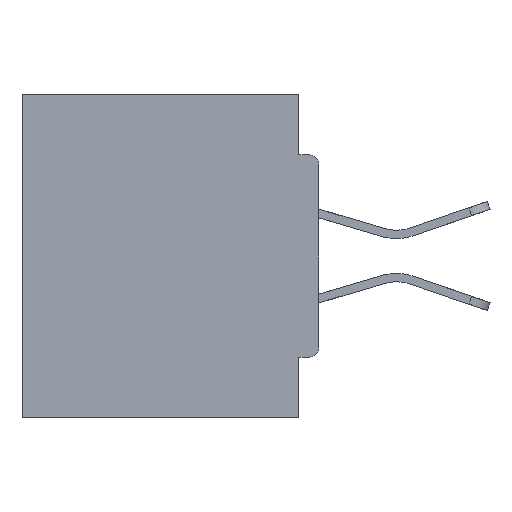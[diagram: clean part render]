
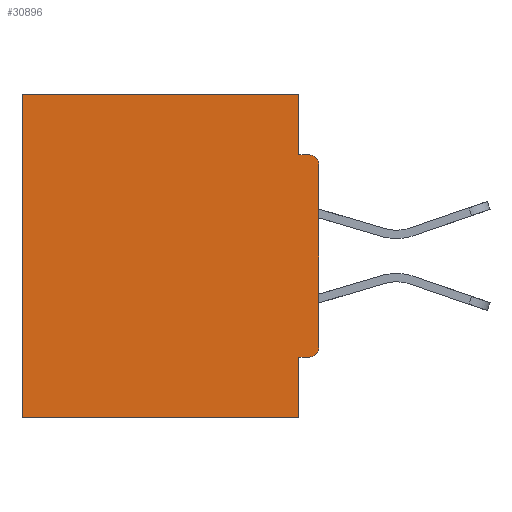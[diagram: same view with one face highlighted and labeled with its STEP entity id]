
A CAD part, left-side view. The second image highlights one B-rep face of the part: STEP entity #30896.
In plain terms, the highlighted planar face has unit normal (-1, 0, 0).
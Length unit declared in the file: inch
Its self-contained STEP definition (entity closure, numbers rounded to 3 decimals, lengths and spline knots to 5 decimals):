
#879 = EDGE_CURVE ( 'NONE', #28704, #24435, #10681, .T. ) ;
#1654 = EDGE_CURVE ( 'NONE', #22127, #19679, #16841, .T. ) ;
#3004 = ORIENTED_EDGE ( 'NONE', *, *, #30974, .F. ) ;
#3491 = DIRECTION ( 'NONE',  ( 0., 0., -1. ) ) ;
#3579 = DIRECTION ( 'NONE',  ( 0., 0., -1. ) ) ;
#3923 = CARTESIAN_POINT ( 'NONE',  ( 0.298, 0.031, -0.5 ) ) ;
#4585 = EDGE_CURVE ( 'NONE', #12120, #24927, #23704, .T. ) ;
#4596 = DIRECTION ( 'NONE',  ( 0., 1., 0. ) ) ;
#5029 = CARTESIAN_POINT ( 'NONE',  ( 0.298, 0.031, -0.5 ) ) ;
#5645 = EDGE_CURVE ( 'NONE', #28704, #21075, #11145, .T. ) ;
#5702 = CARTESIAN_POINT ( 'NONE',  ( 0.298, 0., -0.0935 ) ) ;
#5826 = ORIENTED_EDGE ( 'NONE', *, *, #1654, .F. ) ;
#6322 = CARTESIAN_POINT ( 'NONE',  ( 0.298, 0.031, -0.5 ) ) ;
#6700 = CARTESIAN_POINT ( 'NONE',  ( 0.298, 0., -0.4065 ) ) ;
#6781 = ORIENTED_EDGE ( 'NONE', *, *, #25753, .T. ) ;
#6851 = CARTESIAN_POINT ( 'NONE',  ( 0.298, 0.031, -0.0935 ) ) ;
#6872 = EDGE_CURVE ( 'NONE', #12120, #23094, #12220, .T. ) ;
#6971 = LINE ( 'NONE', #25047, #19478 ) ;
#7345 = DIRECTION ( 'NONE',  ( 0., 0., -1. ) ) ;
#7388 = LINE ( 'NONE', #5702, #29672 ) ;
#7555 = CARTESIAN_POINT ( 'NONE',  ( 0.298, 0.015, -0.4065 ) ) ;
#7778 = DIRECTION ( 'NONE',  ( 0., -1., 0. ) ) ;
#8684 = PLANE ( 'NONE',  #21706 ) ;
#9737 = AXIS2_PLACEMENT_3D ( 'NONE', #18416, #30878, #3491 ) ;
#9887 = VECTOR ( 'NONE', #28281, 39.37008 ) ;
#10078 = CARTESIAN_POINT ( 'NONE',  ( 0.298, 0., -0.1085 ) ) ;
#10387 = CARTESIAN_POINT ( 'NONE',  ( 0.298, 0., 0. ) ) ;
#10681 = LINE ( 'NONE', #10387, #9887 ) ;
#10972 = DIRECTION ( 'NONE',  ( 1., 0., 0. ) ) ;
#11043 = VECTOR ( 'NONE', #21383, 39.37008 ) ;
#11145 = CIRCLE ( 'NONE', #28000, 0.015 ) ;
#12120 = VERTEX_POINT ( 'NONE', #28115 ) ;
#12220 = LINE ( 'NONE', #3923, #11043 ) ;
#12243 = CARTESIAN_POINT ( 'NONE',  ( 0.298, 0.015, -0.1085 ) ) ;
#13390 = CARTESIAN_POINT ( 'NONE',  ( 0.298, 0., 0. ) ) ;
#14209 = ORIENTED_EDGE ( 'NONE', *, *, #5645, .T. ) ;
#15392 = VECTOR ( 'NONE', #3579, 39.37008 ) ;
#15885 = CARTESIAN_POINT ( 'NONE',  ( 0.298, 0.015, -0.0935 ) ) ;
#16770 = CARTESIAN_POINT ( 'NONE',  ( 0.298, 0., 0. ) ) ;
#16841 = LINE ( 'NONE', #6700, #26990 ) ;
#17516 = CARTESIAN_POINT ( 'NONE',  ( 0.298, 0.46, 0. ) ) ;
#18167 = EDGE_CURVE ( 'NONE', #23094, #21075, #7388, .T. ) ;
#18416 = CARTESIAN_POINT ( 'NONE',  ( 0.298, 0.015, -0.3915 ) ) ;
#18737 = DIRECTION ( 'NONE',  ( 0., 0., -1. ) ) ;
#19478 = VECTOR ( 'NONE', #20266, 39.37008 ) ;
#19679 = VERTEX_POINT ( 'NONE', #24096 ) ;
#19708 = ORIENTED_EDGE ( 'NONE', *, *, #29607, .T. ) ;
#20266 = DIRECTION ( 'NONE',  ( 0., 1., 0. ) ) ;
#20270 = VERTEX_POINT ( 'NONE', #5029 ) ;
#20504 = ORIENTED_EDGE ( 'NONE', *, *, #879, .F. ) ;
#20591 = VECTOR ( 'NONE', #26806, 39.37008 ) ;
#21075 = VERTEX_POINT ( 'NONE', #15885 ) ;
#21210 = LINE ( 'NONE', #29680, #23543 ) ;
#21383 = DIRECTION ( 'NONE',  ( 0., 0., -1. ) ) ;
#21706 = AXIS2_PLACEMENT_3D ( 'NONE', #13390, #10972, #18737 ) ;
#22127 = VERTEX_POINT ( 'NONE', #7555 ) ;
#22532 = ORIENTED_EDGE ( 'NONE', *, *, #6872, .F. ) ;
#23094 = VERTEX_POINT ( 'NONE', #6851 ) ;
#23543 = VECTOR ( 'NONE', #27230, 39.37008 ) ;
#23704 = LINE ( 'NONE', #16770, #20591 ) ;
#24096 = CARTESIAN_POINT ( 'NONE',  ( 0.298, 0.031, -0.4065 ) ) ;
#24435 = VERTEX_POINT ( 'NONE', #29015 ) ;
#24927 = VERTEX_POINT ( 'NONE', #17516 ) ;
#25009 = DIRECTION ( 'NONE',  ( -1., 0., 0. ) ) ;
#25047 = CARTESIAN_POINT ( 'NONE',  ( 0.298, 0., -0.5 ) ) ;
#25753 = EDGE_CURVE ( 'NONE', #24927, #26703, #21210, .T. ) ;
#25905 = ORIENTED_EDGE ( 'NONE', *, *, #4585, .T. ) ;
#26703 = VERTEX_POINT ( 'NONE', #31252 ) ;
#26806 = DIRECTION ( 'NONE',  ( 0., 1., 0. ) ) ;
#26990 = VECTOR ( 'NONE', #4596, 39.37008 ) ;
#27230 = DIRECTION ( 'NONE',  ( 0., 0., -1. ) ) ;
#27616 = CIRCLE ( 'NONE', #9737, 0.015 ) ;
#27837 = EDGE_LOOP ( 'NONE', ( #14209, #30251, #22532, #25905, #6781, #32237, #3004, #5826, #19708, #20504 ) ) ;
#27891 = FACE_OUTER_BOUND ( 'NONE', #27837, .T. ) ;
#28000 = AXIS2_PLACEMENT_3D ( 'NONE', #12243, #25009, #7345 ) ;
#28115 = CARTESIAN_POINT ( 'NONE',  ( 0.298, 0.031, 0. ) ) ;
#28281 = DIRECTION ( 'NONE',  ( 0., 0., -1. ) ) ;
#28704 = VERTEX_POINT ( 'NONE', #10078 ) ;
#29015 = CARTESIAN_POINT ( 'NONE',  ( 0.298, 0., -0.3915 ) ) ;
#29077 = EDGE_CURVE ( 'NONE', #20270, #26703, #6971, .T. ) ;
#29607 = EDGE_CURVE ( 'NONE', #22127, #24435, #27616, .T. ) ;
#29672 = VECTOR ( 'NONE', #7778, 39.37008 ) ;
#29680 = CARTESIAN_POINT ( 'NONE',  ( 0.298, 0.46, 0. ) ) ;
#30251 = ORIENTED_EDGE ( 'NONE', *, *, #18167, .F. ) ;
#30260 = LINE ( 'NONE', #6322, #15392 ) ;
#30878 = DIRECTION ( 'NONE',  ( -1., 0., 0. ) ) ;
#30896 = ADVANCED_FACE ( 'NONE', ( #27891 ), #8684, .F. ) ;
#30974 = EDGE_CURVE ( 'NONE', #19679, #20270, #30260, .T. ) ;
#31252 = CARTESIAN_POINT ( 'NONE',  ( 0.298, 0.46, -0.5 ) ) ;
#32237 = ORIENTED_EDGE ( 'NONE', *, *, #29077, .F. ) ;
